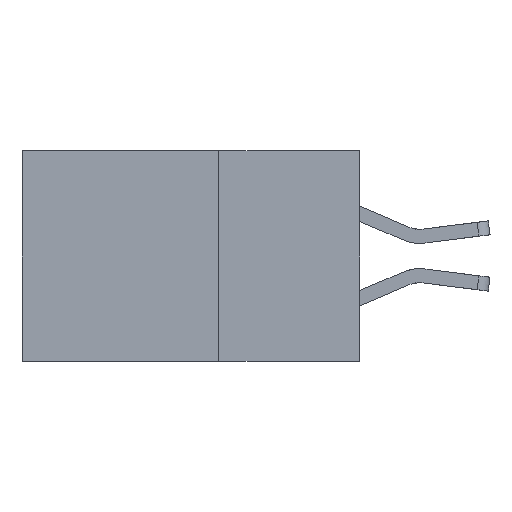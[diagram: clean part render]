
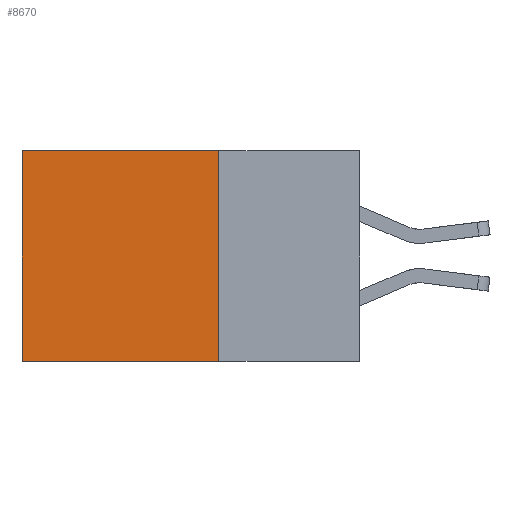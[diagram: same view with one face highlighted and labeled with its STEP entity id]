
A CAD part, left-side view. The second image highlights one B-rep face of the part: STEP entity #8670.
In plain terms, the highlighted planar face has unit normal (-1, 0, 0).
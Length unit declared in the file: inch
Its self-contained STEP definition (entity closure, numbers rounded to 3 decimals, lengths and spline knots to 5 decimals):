
#85 = CARTESIAN_POINT ( 'NONE',  ( 0.2875, 0.6, 0. ) ) ;
#158 = CARTESIAN_POINT ( 'NONE',  ( 0.2875, 0.25, 0. ) ) ;
#249 = PLANE ( 'NONE',  #6197 ) ;
#891 = LINE ( 'NONE', #8765, #5805 ) ;
#987 = CARTESIAN_POINT ( 'NONE',  ( 0.2875, 0.6, -0.375 ) ) ;
#1032 = VERTEX_POINT ( 'NONE', #987 ) ;
#1110 = EDGE_CURVE ( 'NONE', #7224, #8776, #891, .T. ) ;
#1973 = DIRECTION ( 'NONE',  ( 0., 0., -1. ) ) ;
#2014 = CARTESIAN_POINT ( 'NONE',  ( 0.2875, 0.6, -0.375 ) ) ;
#2233 = ORIENTED_EDGE ( 'NONE', *, *, #5553, .T. ) ;
#2243 = DIRECTION ( 'NONE',  ( 0., 1., 0. ) ) ;
#2282 = CARTESIAN_POINT ( 'NONE',  ( 0.2875, 0.25, -0.375 ) ) ;
#3095 = ORIENTED_EDGE ( 'NONE', *, *, #5030, .T. ) ;
#3690 = DIRECTION ( 'NONE',  ( 0., 0., -1. ) ) ;
#4778 = VECTOR ( 'NONE', #5591, 39.37008 ) ;
#4989 = ORIENTED_EDGE ( 'NONE', *, *, #1110, .F. ) ;
#5025 = CARTESIAN_POINT ( 'NONE',  ( 0.2875, 0.25, -0.375 ) ) ;
#5030 = EDGE_CURVE ( 'NONE', #7020, #1032, #7178, .T. ) ;
#5037 = VECTOR ( 'NONE', #2243, 39.37008 ) ;
#5043 = CARTESIAN_POINT ( 'NONE',  ( 0.2875, 0.25, 0. ) ) ;
#5150 = ORIENTED_EDGE ( 'NONE', *, *, #6744, .F. ) ;
#5357 = DIRECTION ( 'NONE',  ( 0., 0., -1. ) ) ;
#5457 = CARTESIAN_POINT ( 'NONE',  ( 0.2875, 0.25, -0.375 ) ) ;
#5494 = EDGE_LOOP ( 'NONE', ( #3095, #5150, #4989, #2233 ) ) ;
#5553 = EDGE_CURVE ( 'NONE', #7224, #7020, #6199, .T. ) ;
#5591 = DIRECTION ( 'NONE',  ( 0., 1., 0. ) ) ;
#5805 = VECTOR ( 'NONE', #1973, 39.37008 ) ;
#5840 = FACE_OUTER_BOUND ( 'NONE', #5494, .T. ) ;
#6197 = AXIS2_PLACEMENT_3D ( 'NONE', #5025, #7767, #3690 ) ;
#6199 = LINE ( 'NONE', #5043, #5037 ) ;
#6744 = EDGE_CURVE ( 'NONE', #8776, #1032, #7459, .T. ) ;
#7020 = VERTEX_POINT ( 'NONE', #85 ) ;
#7178 = LINE ( 'NONE', #2014, #8020 ) ;
#7224 = VERTEX_POINT ( 'NONE', #158 ) ;
#7459 = LINE ( 'NONE', #2282, #4778 ) ;
#7767 = DIRECTION ( 'NONE',  ( 1., 0., 0. ) ) ;
#8020 = VECTOR ( 'NONE', #5357, 39.37008 ) ;
#8670 = ADVANCED_FACE ( 'NONE', ( #5840 ), #249, .F. ) ;
#8765 = CARTESIAN_POINT ( 'NONE',  ( 0.2875, 0.25, -0.375 ) ) ;
#8776 = VERTEX_POINT ( 'NONE', #5457 ) ;
